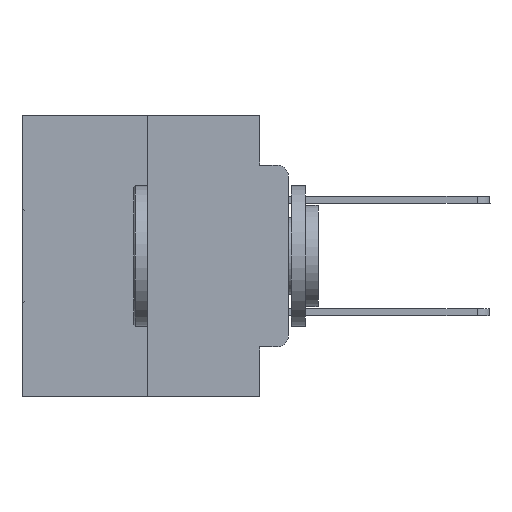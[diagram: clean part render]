
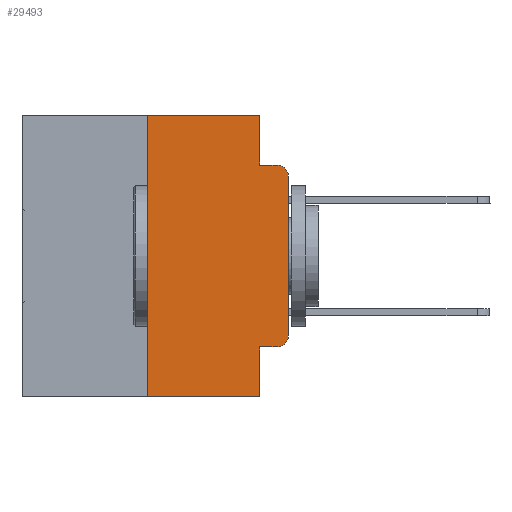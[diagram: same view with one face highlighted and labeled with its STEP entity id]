
A CAD part, left-side view. The second image highlights one B-rep face of the part: STEP entity #29493.
In plain terms, the highlighted planar face has unit normal (-1, 0, 0).
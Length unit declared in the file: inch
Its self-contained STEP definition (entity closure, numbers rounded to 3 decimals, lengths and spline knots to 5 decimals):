
#1107 = VERTEX_POINT ( 'NONE', #15914 ) ;
#1273 = CARTESIAN_POINT ( 'NONE',  ( 0., 0.25, 0. ) ) ;
#1601 = CARTESIAN_POINT ( 'NONE',  ( 0., 0.051, -0.0885 ) ) ;
#2041 = VERTEX_POINT ( 'NONE', #16315 ) ;
#2884 = ORIENTED_EDGE ( 'NONE', *, *, #22421, .T. ) ;
#3320 = EDGE_CURVE ( 'NONE', #25661, #1107, #10801, .T. ) ;
#3481 = CIRCLE ( 'NONE', #21740, 0.02 ) ;
#3680 = CIRCLE ( 'NONE', #6830, 0.02 ) ;
#4280 = ORIENTED_EDGE ( 'NONE', *, *, #3320, .F. ) ;
#4699 = DIRECTION ( 'NONE',  ( 0., 0., -1. ) ) ;
#4854 = VECTOR ( 'NONE', #26668, 39.37008 ) ;
#5208 = VECTOR ( 'NONE', #5816, 39.37008 ) ;
#5396 = EDGE_CURVE ( 'NONE', #18129, #28232, #21684, .T. ) ;
#5567 = CARTESIAN_POINT ( 'NONE',  ( 0., 0.02, -0.3915 ) ) ;
#5575 = CARTESIAN_POINT ( 'NONE',  ( 0., 0.473, -0.5 ) ) ;
#5816 = DIRECTION ( 'NONE',  ( 0., -1., 0. ) ) ;
#6348 = EDGE_CURVE ( 'NONE', #2041, #8372, #28034, .T. ) ;
#6830 = AXIS2_PLACEMENT_3D ( 'NONE', #15058, #7848, #25007 ) ;
#6978 = DIRECTION ( 'NONE',  ( 0., -1., 0. ) ) ;
#7232 = CARTESIAN_POINT ( 'NONE',  ( 0., 0.473, 0. ) ) ;
#7568 = ORIENTED_EDGE ( 'NONE', *, *, #7839, .F. ) ;
#7839 = EDGE_CURVE ( 'NONE', #27730, #26431, #14810, .T. ) ;
#7848 = DIRECTION ( 'NONE',  ( -1., 0., 0. ) ) ;
#8183 = CARTESIAN_POINT ( 'NONE',  ( 0., 0.051, -0.4115 ) ) ;
#8199 = CARTESIAN_POINT ( 'NONE',  ( 0., 0., -0.1085 ) ) ;
#8372 = VERTEX_POINT ( 'NONE', #8199 ) ;
#8574 = ORIENTED_EDGE ( 'NONE', *, *, #27705, .T. ) ;
#8775 = ORIENTED_EDGE ( 'NONE', *, *, #27770, .T. ) ;
#10499 = EDGE_LOOP ( 'NONE', ( #22537, #8775, #20827, #28331, #27176, #7568, #8574, #4280, #30659, #2884 ) ) ;
#10801 = LINE ( 'NONE', #23833, #25026 ) ;
#11595 = CARTESIAN_POINT ( 'NONE',  ( 0., 0.02, -0.0885 ) ) ;
#11963 = LINE ( 'NONE', #7232, #4854 ) ;
#12755 = DIRECTION ( 'NONE',  ( 0., 0., -1. ) ) ;
#13265 = CARTESIAN_POINT ( 'NONE',  ( 0., 0.25, -0.5 ) ) ;
#14732 = AXIS2_PLACEMENT_3D ( 'NONE', #25935, #21525, #18431 ) ;
#14810 = LINE ( 'NONE', #31957, #16675 ) ;
#15058 = CARTESIAN_POINT ( 'NONE',  ( 0., 0.02, -0.1085 ) ) ;
#15634 = CARTESIAN_POINT ( 'NONE',  ( 0., 0., 0. ) ) ;
#15914 = CARTESIAN_POINT ( 'NONE',  ( 0., 0.051, -0.5 ) ) ;
#16315 = CARTESIAN_POINT ( 'NONE',  ( 0., 0., -0.3915 ) ) ;
#16460 = PLANE ( 'NONE',  #14732 ) ;
#16675 = VECTOR ( 'NONE', #19874, 39.37008 ) ;
#17222 = CARTESIAN_POINT ( 'NONE',  ( 0., 0.02, -0.4115 ) ) ;
#18129 = VERTEX_POINT ( 'NONE', #22440 ) ;
#18396 = EDGE_CURVE ( 'NONE', #26431, #18129, #11963, .T. ) ;
#18431 = DIRECTION ( 'NONE',  ( 0., 0., -1. ) ) ;
#19364 = CARTESIAN_POINT ( 'NONE',  ( 0., 0.051, -0.0885 ) ) ;
#19874 = DIRECTION ( 'NONE',  ( 0., 0., 1. ) ) ;
#20827 = ORIENTED_EDGE ( 'NONE', *, *, #23246, .F. ) ;
#21075 = DIRECTION ( 'NONE',  ( 0., 0., -1. ) ) ;
#21525 = DIRECTION ( 'NONE',  ( 1., 0., 0. ) ) ;
#21684 = LINE ( 'NONE', #24609, #22222 ) ;
#21740 = AXIS2_PLACEMENT_3D ( 'NONE', #5567, #27933, #12755 ) ;
#22222 = VECTOR ( 'NONE', #4699, 39.37008 ) ;
#22421 = EDGE_CURVE ( 'NONE', #27052, #2041, #3481, .T. ) ;
#22440 = CARTESIAN_POINT ( 'NONE',  ( 0., 0.051, 0. ) ) ;
#22537 = ORIENTED_EDGE ( 'NONE', *, *, #6348, .T. ) ;
#23246 = EDGE_CURVE ( 'NONE', #28232, #32130, #29357, .T. ) ;
#23833 = CARTESIAN_POINT ( 'NONE',  ( 0., 0.051, 0. ) ) ;
#24012 = VECTOR ( 'NONE', #25662, 39.37008 ) ;
#24609 = CARTESIAN_POINT ( 'NONE',  ( 0., 0.051, 0. ) ) ;
#25007 = DIRECTION ( 'NONE',  ( 0., 0., -1. ) ) ;
#25026 = VECTOR ( 'NONE', #21075, 39.37008 ) ;
#25063 = VECTOR ( 'NONE', #25597, 39.37008 ) ;
#25597 = DIRECTION ( 'NONE',  ( 0., 0., 1. ) ) ;
#25661 = VERTEX_POINT ( 'NONE', #8183 ) ;
#25662 = DIRECTION ( 'NONE',  ( 0., -1., 0. ) ) ;
#25935 = CARTESIAN_POINT ( 'NONE',  ( 0., 0.473, 0. ) ) ;
#26431 = VERTEX_POINT ( 'NONE', #1273 ) ;
#26668 = DIRECTION ( 'NONE',  ( 0., -1., 0. ) ) ;
#26716 = EDGE_CURVE ( 'NONE', #25661, #27052, #29672, .T. ) ;
#27019 = VECTOR ( 'NONE', #6978, 39.37008 ) ;
#27052 = VERTEX_POINT ( 'NONE', #17222 ) ;
#27176 = ORIENTED_EDGE ( 'NONE', *, *, #18396, .F. ) ;
#27705 = EDGE_CURVE ( 'NONE', #27730, #1107, #30238, .T. ) ;
#27730 = VERTEX_POINT ( 'NONE', #13265 ) ;
#27770 = EDGE_CURVE ( 'NONE', #8372, #32130, #3680, .T. ) ;
#27933 = DIRECTION ( 'NONE',  ( -1., 0., 0. ) ) ;
#28034 = LINE ( 'NONE', #15634, #25063 ) ;
#28232 = VERTEX_POINT ( 'NONE', #19364 ) ;
#28331 = ORIENTED_EDGE ( 'NONE', *, *, #5396, .F. ) ;
#28698 = FACE_OUTER_BOUND ( 'NONE', #10499, .T. ) ;
#29357 = LINE ( 'NONE', #1601, #27019 ) ;
#29493 = ADVANCED_FACE ( 'NONE', ( #28698 ), #16460, .F. ) ;
#29672 = LINE ( 'NONE', #30631, #5208 ) ;
#30238 = LINE ( 'NONE', #5575, #24012 ) ;
#30631 = CARTESIAN_POINT ( 'NONE',  ( 0., 0.051, -0.4115 ) ) ;
#30659 = ORIENTED_EDGE ( 'NONE', *, *, #26716, .T. ) ;
#31957 = CARTESIAN_POINT ( 'NONE',  ( 0., 0.25, 0. ) ) ;
#32130 = VERTEX_POINT ( 'NONE', #11595 ) ;
